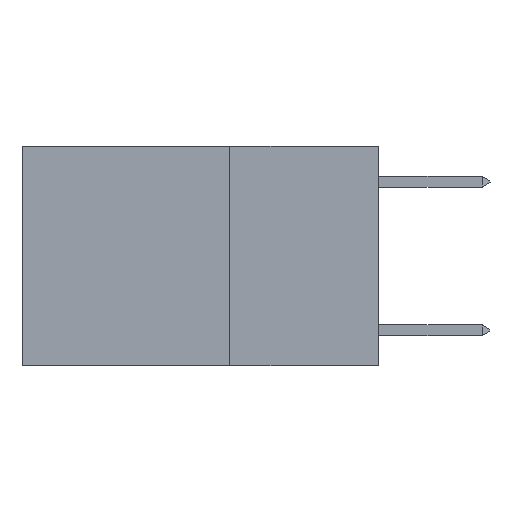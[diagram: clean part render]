
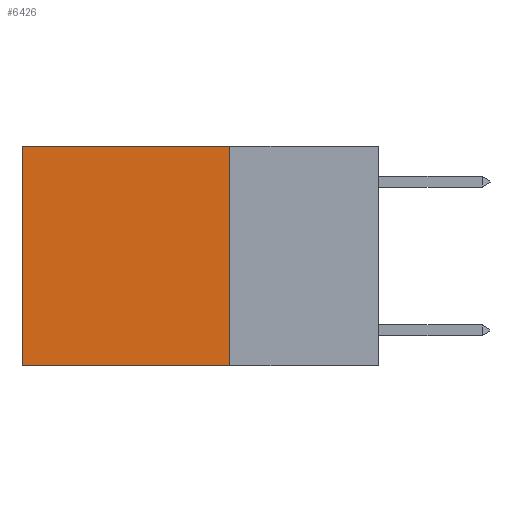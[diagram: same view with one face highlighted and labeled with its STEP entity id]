
A CAD part, left-side view. The second image highlights one B-rep face of the part: STEP entity #6426.
In plain terms, the highlighted planar face has unit normal (-1, 0, 0).
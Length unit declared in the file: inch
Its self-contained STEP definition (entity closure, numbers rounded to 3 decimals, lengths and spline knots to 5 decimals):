
#404 = DIRECTION ( 'NONE',  ( 1., 0., 0. ) ) ;
#1001 = VERTEX_POINT ( 'NONE', #5881 ) ;
#1074 = VECTOR ( 'NONE', #11497, 39.37008 ) ;
#1101 = ORIENTED_EDGE ( 'NONE', *, *, #15592, .F. ) ;
#1380 = CARTESIAN_POINT ( 'NONE',  ( 0.2625, 0.25, 0. ) ) ;
#1611 = ORIENTED_EDGE ( 'NONE', *, *, #13820, .T. ) ;
#2008 = EDGE_LOOP ( 'NONE', ( #1611, #1101, #6047, #2806 ) ) ;
#2487 = CARTESIAN_POINT ( 'NONE',  ( 0.2625, 0.6, -0.37 ) ) ;
#2806 = ORIENTED_EDGE ( 'NONE', *, *, #10297, .T. ) ;
#2960 = CARTESIAN_POINT ( 'NONE',  ( 0.2625, 0.6, 0. ) ) ;
#3110 = CARTESIAN_POINT ( 'NONE',  ( 0.2625, 0.6, 0. ) ) ;
#3211 = VECTOR ( 'NONE', #10732, 39.37008 ) ;
#3604 = LINE ( 'NONE', #2960, #3211 ) ;
#4414 = LINE ( 'NONE', #1380, #14272 ) ;
#4522 = LINE ( 'NONE', #8949, #1074 ) ;
#4675 = EDGE_CURVE ( 'NONE', #1001, #14099, #4414, .T. ) ;
#5279 = VERTEX_POINT ( 'NONE', #2487 ) ;
#5624 = VERTEX_POINT ( 'NONE', #3110 ) ;
#5881 = CARTESIAN_POINT ( 'NONE',  ( 0.2625, 0.25, 0. ) ) ;
#6011 = VECTOR ( 'NONE', #6201, 39.37008 ) ;
#6047 = ORIENTED_EDGE ( 'NONE', *, *, #4675, .F. ) ;
#6201 = DIRECTION ( 'NONE',  ( 0., 1., 0. ) ) ;
#6426 = ADVANCED_FACE ( 'NONE', ( #16241 ), #14548, .F. ) ;
#8232 = CARTESIAN_POINT ( 'NONE',  ( 0.2625, 0.25, 0. ) ) ;
#8949 = CARTESIAN_POINT ( 'NONE',  ( 0.2625, 0.25, 0. ) ) ;
#9500 = DIRECTION ( 'NONE',  ( 0., 0., -1. ) ) ;
#10297 = EDGE_CURVE ( 'NONE', #1001, #5624, #4522, .T. ) ;
#10732 = DIRECTION ( 'NONE',  ( 0., 0., -1. ) ) ;
#11497 = DIRECTION ( 'NONE',  ( 0., 1., 0. ) ) ;
#11732 = DIRECTION ( 'NONE',  ( 0., 0., -1. ) ) ;
#13780 = CARTESIAN_POINT ( 'NONE',  ( 0.2625, 0.25, -0.37 ) ) ;
#13820 = EDGE_CURVE ( 'NONE', #5624, #5279, #3604, .T. ) ;
#14010 = AXIS2_PLACEMENT_3D ( 'NONE', #8232, #404, #9500 ) ;
#14099 = VERTEX_POINT ( 'NONE', #13780 ) ;
#14272 = VECTOR ( 'NONE', #11732, 39.37008 ) ;
#14548 = PLANE ( 'NONE',  #14010 ) ;
#15592 = EDGE_CURVE ( 'NONE', #14099, #5279, #15842, .T. ) ;
#15842 = LINE ( 'NONE', #16448, #6011 ) ;
#16241 = FACE_OUTER_BOUND ( 'NONE', #2008, .T. ) ;
#16448 = CARTESIAN_POINT ( 'NONE',  ( 0.2625, 0.25, -0.37 ) ) ;
